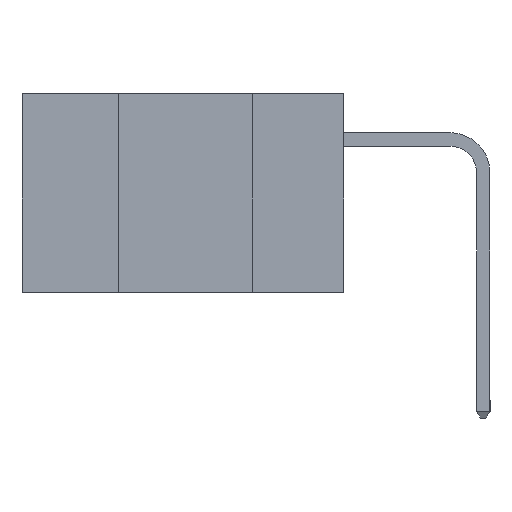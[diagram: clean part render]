
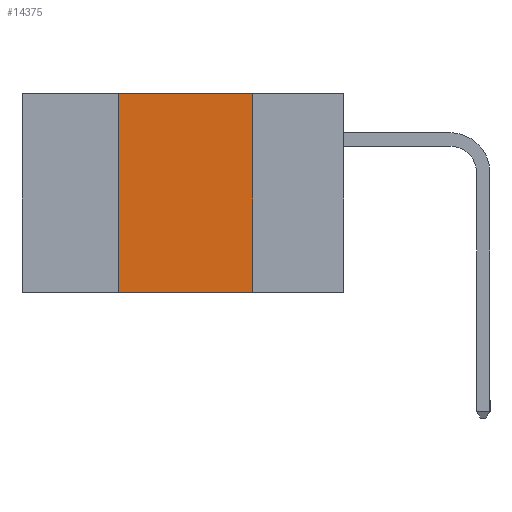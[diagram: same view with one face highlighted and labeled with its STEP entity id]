
A CAD part, left-side view. The second image highlights one B-rep face of the part: STEP entity #14375.
In plain terms, the highlighted planar face has unit normal (-1, 0, 0).
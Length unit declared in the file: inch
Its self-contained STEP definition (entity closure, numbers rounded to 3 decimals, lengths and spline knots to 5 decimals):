
#238 = DIRECTION ( 'NONE',  ( 0., -1., 0. ) ) ;
#574 = EDGE_CURVE ( 'NONE', #13334, #14148, #1623, .T. ) ;
#776 = CARTESIAN_POINT ( 'NONE',  ( 0., 0.17, 0. ) ) ;
#1453 = VERTEX_POINT ( 'NONE', #776 ) ;
#1537 = EDGE_CURVE ( 'NONE', #13334, #10118, #7819, .T. ) ;
#1623 = LINE ( 'NONE', #11778, #5155 ) ;
#3154 = DIRECTION ( 'NONE',  ( 0., 0., 1. ) ) ;
#3496 = FACE_OUTER_BOUND ( 'NONE', #13919, .T. ) ;
#3591 = PLANE ( 'NONE',  #5583 ) ;
#3849 = EDGE_CURVE ( 'NONE', #14148, #1453, #10668, .T. ) ;
#5075 = CARTESIAN_POINT ( 'NONE',  ( 0., 0.17, -0.37 ) ) ;
#5155 = VECTOR ( 'NONE', #3154, 39.37008 ) ;
#5583 = AXIS2_PLACEMENT_3D ( 'NONE', #9299, #5966, #13683 ) ;
#5910 = ORIENTED_EDGE ( 'NONE', *, *, #1537, .T. ) ;
#5966 = DIRECTION ( 'NONE',  ( 1., 0., 0. ) ) ;
#6641 = ORIENTED_EDGE ( 'NONE', *, *, #3849, .F. ) ;
#7138 = VECTOR ( 'NONE', #12893, 39.37008 ) ;
#7819 = LINE ( 'NONE', #14552, #10438 ) ;
#8930 = CARTESIAN_POINT ( 'NONE',  ( 0., 0.42, 0. ) ) ;
#9247 = ORIENTED_EDGE ( 'NONE', *, *, #574, .F. ) ;
#9299 = CARTESIAN_POINT ( 'NONE',  ( 0., 0.6, 0. ) ) ;
#10028 = CARTESIAN_POINT ( 'NONE',  ( 0., 0.6, 0. ) ) ;
#10104 = DIRECTION ( 'NONE',  ( 0., -1., 0. ) ) ;
#10116 = LINE ( 'NONE', #5075, #7138 ) ;
#10118 = VERTEX_POINT ( 'NONE', #11139 ) ;
#10438 = VECTOR ( 'NONE', #238, 39.37008 ) ;
#10668 = LINE ( 'NONE', #10028, #13215 ) ;
#11139 = CARTESIAN_POINT ( 'NONE',  ( 0., 0.17, -0.37 ) ) ;
#11778 = CARTESIAN_POINT ( 'NONE',  ( 0., 0.42, -0.37 ) ) ;
#12497 = ORIENTED_EDGE ( 'NONE', *, *, #14521, .F. ) ;
#12513 = CARTESIAN_POINT ( 'NONE',  ( 0., 0.42, -0.37 ) ) ;
#12893 = DIRECTION ( 'NONE',  ( 0., 0., -1. ) ) ;
#13215 = VECTOR ( 'NONE', #10104, 39.37008 ) ;
#13334 = VERTEX_POINT ( 'NONE', #12513 ) ;
#13683 = DIRECTION ( 'NONE',  ( 0., 0., -1. ) ) ;
#13919 = EDGE_LOOP ( 'NONE', ( #12497, #6641, #9247, #5910 ) ) ;
#14148 = VERTEX_POINT ( 'NONE', #8930 ) ;
#14375 = ADVANCED_FACE ( 'NONE', ( #3496 ), #3591, .F. ) ;
#14521 = EDGE_CURVE ( 'NONE', #1453, #10118, #10116, .T. ) ;
#14552 = CARTESIAN_POINT ( 'NONE',  ( 0., 0.6, -0.37 ) ) ;
